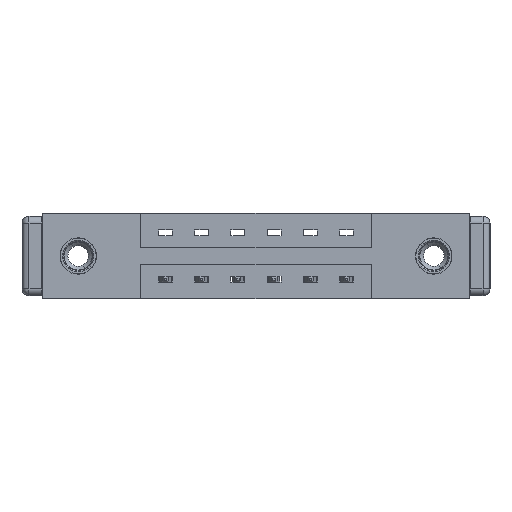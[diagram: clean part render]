
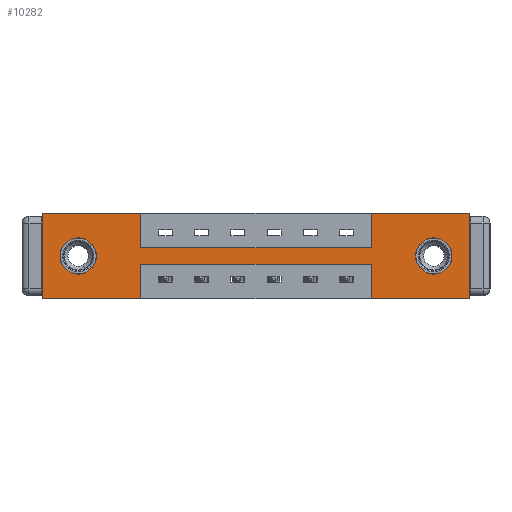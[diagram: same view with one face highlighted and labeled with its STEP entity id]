
A CAD part, front view. The second image highlights one B-rep face of the part: STEP entity #10282.
In plain terms, the highlighted planar face has unit normal (0, -1, 0).
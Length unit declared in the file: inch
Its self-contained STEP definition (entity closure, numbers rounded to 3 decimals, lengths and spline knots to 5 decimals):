
#46 = VERTEX_POINT ( 'NONE', #573 ) ;
#138 = DIRECTION ( 'NONE',  ( 0., -1., 0. ) ) ;
#160 = LINE ( 'NONE', #326, #3913 ) ;
#166 = DIRECTION ( 'NONE',  ( 0., 0., -1. ) ) ;
#237 = DIRECTION ( 'NONE',  ( -1., 0., 0. ) ) ;
#245 = VECTOR ( 'NONE', #1814, 39.37008 ) ;
#326 = CARTESIAN_POINT ( 'NONE',  ( 0.425, 0., 0. ) ) ;
#418 = ORIENTED_EDGE ( 'NONE', *, *, #6473, .F. ) ;
#452 = DIRECTION ( 'NONE',  ( 0., 0., 1. ) ) ;
#557 = VECTOR ( 'NONE', #10802, 39.37008 ) ;
#563 = DIRECTION ( 'NONE',  ( 1., 0., 0. ) ) ;
#570 = FACE_OUTER_BOUND ( 'NONE', #8843, .T. ) ;
#573 = CARTESIAN_POINT ( 'NONE',  ( 1.842, 0., -0.37 ) ) ;
#594 = EDGE_CURVE ( 'NONE', #11487, #4366, #7277, .T. ) ;
#662 = CARTESIAN_POINT ( 'NONE',  ( 1.417, 0., 0. ) ) ;
#727 = LINE ( 'NONE', #2094, #2182 ) ;
#768 = CARTESIAN_POINT ( 'NONE',  ( 0., 0., -0.37 ) ) ;
#1134 = ORIENTED_EDGE ( 'NONE', *, *, #7737, .T. ) ;
#1245 = CARTESIAN_POINT ( 'NONE',  ( 0., 0., -0.37 ) ) ;
#1270 = VERTEX_POINT ( 'NONE', #10253 ) ;
#1301 = CARTESIAN_POINT ( 'NONE',  ( 0.155, 0., -0.107 ) ) ;
#1448 = EDGE_CURVE ( 'NONE', #4177, #11317, #9568, .T. ) ;
#1537 = CIRCLE ( 'NONE', #11228, 0.078 ) ;
#1570 = CARTESIAN_POINT ( 'NONE',  ( 0.155, 0., -0.185 ) ) ;
#1618 = VECTOR ( 'NONE', #10195, 39.37008 ) ;
#1705 = VECTOR ( 'NONE', #9914, 39.37008 ) ;
#1814 = DIRECTION ( 'NONE',  ( 0., 0., -1. ) ) ;
#1933 = DIRECTION ( 'NONE',  ( 1., 0., 0. ) ) ;
#2000 = DIRECTION ( 'NONE',  ( 0., 0., -1. ) ) ;
#2094 = CARTESIAN_POINT ( 'NONE',  ( 0.425, 0., -0.22 ) ) ;
#2120 = EDGE_CURVE ( 'NONE', #9738, #4177, #160, .T. ) ;
#2182 = VECTOR ( 'NONE', #237, 39.37008 ) ;
#2196 = LINE ( 'NONE', #4345, #9953 ) ;
#2490 = DIRECTION ( 'NONE',  ( 0., 1., 0. ) ) ;
#2588 = CARTESIAN_POINT ( 'NONE',  ( 1.417, 0., -0.15 ) ) ;
#2701 = AXIS2_PLACEMENT_3D ( 'NONE', #9938, #4414, #6183 ) ;
#2781 = CARTESIAN_POINT ( 'NONE',  ( 0.425, 0., -0.37 ) ) ;
#2859 = VECTOR ( 'NONE', #11718, 39.37008 ) ;
#2894 = CIRCLE ( 'NONE', #2701, 0.078 ) ;
#2945 = ORIENTED_EDGE ( 'NONE', *, *, #6117, .F. ) ;
#3009 = FACE_BOUND ( 'NONE', #6900, .T. ) ;
#3201 = VERTEX_POINT ( 'NONE', #9277 ) ;
#3442 = EDGE_CURVE ( 'NONE', #6427, #46, #11094, .T. ) ;
#3614 = CARTESIAN_POINT ( 'NONE',  ( 0., 0., 0. ) ) ;
#3913 = VECTOR ( 'NONE', #166, 39.37008 ) ;
#3987 = CARTESIAN_POINT ( 'NONE',  ( 1.417, 0., 0. ) ) ;
#4002 = CARTESIAN_POINT ( 'NONE',  ( 0., 0., -0.37 ) ) ;
#4124 = ORIENTED_EDGE ( 'NONE', *, *, #594, .T. ) ;
#4177 = VERTEX_POINT ( 'NONE', #4698 ) ;
#4199 = ORIENTED_EDGE ( 'NONE', *, *, #7812, .T. ) ;
#4278 = CARTESIAN_POINT ( 'NONE',  ( 0.425, 0., -0.22 ) ) ;
#4290 = CARTESIAN_POINT ( 'NONE',  ( 0.155, 0., -0.185 ) ) ;
#4345 = CARTESIAN_POINT ( 'NONE',  ( 0., 0., 0. ) ) ;
#4366 = VERTEX_POINT ( 'NONE', #5213 ) ;
#4414 = DIRECTION ( 'NONE',  ( 0., 1., 0. ) ) ;
#4698 = CARTESIAN_POINT ( 'NONE',  ( 0.425, 0., -0.15 ) ) ;
#4925 = EDGE_CURVE ( 'NONE', #46, #6889, #5224, .T. ) ;
#4949 = CARTESIAN_POINT ( 'NONE',  ( 0.425, 0., -0.37 ) ) ;
#4983 = VECTOR ( 'NONE', #6867, 39.37008 ) ;
#5023 = EDGE_CURVE ( 'NONE', #8351, #9299, #7412, .T. ) ;
#5213 = CARTESIAN_POINT ( 'NONE',  ( 1.687, 0., -0.107 ) ) ;
#5224 = LINE ( 'NONE', #768, #6534 ) ;
#5279 = CIRCLE ( 'NONE', #10383, 0.078 ) ;
#5541 = CARTESIAN_POINT ( 'NONE',  ( 0.425, 0., 0. ) ) ;
#5774 = ORIENTED_EDGE ( 'NONE', *, *, #7028, .F. ) ;
#5813 = EDGE_CURVE ( 'NONE', #4366, #11487, #2894, .T. ) ;
#5886 = ORIENTED_EDGE ( 'NONE', *, *, #3442, .F. ) ;
#6117 = EDGE_CURVE ( 'NONE', #9299, #9738, #2196, .T. ) ;
#6183 = DIRECTION ( 'NONE',  ( 0., 0., -1. ) ) ;
#6295 = EDGE_CURVE ( 'NONE', #3201, #9210, #727, .T. ) ;
#6316 = LINE ( 'NONE', #662, #1705 ) ;
#6383 = VECTOR ( 'NONE', #8761, 39.37008 ) ;
#6427 = VERTEX_POINT ( 'NONE', #9711 ) ;
#6443 = LINE ( 'NONE', #1245, #4983 ) ;
#6473 = EDGE_CURVE ( 'NONE', #7090, #6427, #10975, .T. ) ;
#6534 = VECTOR ( 'NONE', #8065, 39.37008 ) ;
#6540 = ORIENTED_EDGE ( 'NONE', *, *, #5023, .F. ) ;
#6567 = DIRECTION ( 'NONE',  ( 0., 1., 0. ) ) ;
#6658 = ORIENTED_EDGE ( 'NONE', *, *, #8107, .F. ) ;
#6688 = ORIENTED_EDGE ( 'NONE', *, *, #6295, .F. ) ;
#6783 = ORIENTED_EDGE ( 'NONE', *, *, #4925, .F. ) ;
#6867 = DIRECTION ( 'NONE',  ( -1., 0., 0. ) ) ;
#6889 = VERTEX_POINT ( 'NONE', #10578 ) ;
#6900 = EDGE_LOOP ( 'NONE', ( #4199, #1134 ) ) ;
#6918 = LINE ( 'NONE', #8173, #2859 ) ;
#7028 = EDGE_CURVE ( 'NONE', #11317, #7090, #6316, .T. ) ;
#7090 = VERTEX_POINT ( 'NONE', #3987 ) ;
#7247 = PLANE ( 'NONE',  #9164 ) ;
#7277 = CIRCLE ( 'NONE', #7727, 0.078 ) ;
#7412 = LINE ( 'NONE', #3614, #1618 ) ;
#7420 = DIRECTION ( 'NONE',  ( 0., 0., -1. ) ) ;
#7431 = VERTEX_POINT ( 'NONE', #1301 ) ;
#7483 = EDGE_LOOP ( 'NONE', ( #7534, #4124 ) ) ;
#7534 = ORIENTED_EDGE ( 'NONE', *, *, #5813, .T. ) ;
#7586 = CARTESIAN_POINT ( 'NONE',  ( 1.687, 0., -0.185 ) ) ;
#7622 = LINE ( 'NONE', #2781, #245 ) ;
#7727 = AXIS2_PLACEMENT_3D ( 'NONE', #7586, #6567, #7420 ) ;
#7737 = EDGE_CURVE ( 'NONE', #1270, #7431, #1537, .T. ) ;
#7812 = EDGE_CURVE ( 'NONE', #7431, #1270, #5279, .T. ) ;
#7943 = FACE_BOUND ( 'NONE', #7483, .T. ) ;
#7944 = EDGE_CURVE ( 'NONE', #9210, #9066, #7622, .T. ) ;
#7955 = ORIENTED_EDGE ( 'NONE', *, *, #11309, .F. ) ;
#8065 = DIRECTION ( 'NONE',  ( -1., 0., 0. ) ) ;
#8107 = EDGE_CURVE ( 'NONE', #9066, #8351, #6443, .T. ) ;
#8173 = CARTESIAN_POINT ( 'NONE',  ( 1.417, 0., -0.37 ) ) ;
#8182 = CARTESIAN_POINT ( 'NONE',  ( 0., 0., -0.37 ) ) ;
#8351 = VERTEX_POINT ( 'NONE', #4002 ) ;
#8479 = ORIENTED_EDGE ( 'NONE', *, *, #2120, .F. ) ;
#8485 = ORIENTED_EDGE ( 'NONE', *, *, #1448, .F. ) ;
#8534 = VECTOR ( 'NONE', #1933, 39.37008 ) ;
#8761 = DIRECTION ( 'NONE',  ( 1., 0., 0. ) ) ;
#8843 = EDGE_LOOP ( 'NONE', ( #11844, #6688, #7955, #6783, #5886, #418, #5774, #8485, #8479, #2945, #6540, #6658 ) ) ;
#9066 = VERTEX_POINT ( 'NONE', #4949 ) ;
#9164 = AXIS2_PLACEMENT_3D ( 'NONE', #8182, #138, #2000 ) ;
#9210 = VERTEX_POINT ( 'NONE', #4278 ) ;
#9277 = CARTESIAN_POINT ( 'NONE',  ( 1.417, 0., -0.22 ) ) ;
#9299 = VERTEX_POINT ( 'NONE', #10990 ) ;
#9568 = LINE ( 'NONE', #11471, #6383 ) ;
#9711 = CARTESIAN_POINT ( 'NONE',  ( 1.842, 0., 0. ) ) ;
#9738 = VERTEX_POINT ( 'NONE', #5541 ) ;
#9852 = CARTESIAN_POINT ( 'NONE',  ( 1.842, 0., 0. ) ) ;
#9914 = DIRECTION ( 'NONE',  ( 0., 0., 1. ) ) ;
#9938 = CARTESIAN_POINT ( 'NONE',  ( 1.687, 0., -0.185 ) ) ;
#9953 = VECTOR ( 'NONE', #563, 39.37008 ) ;
#10195 = DIRECTION ( 'NONE',  ( 0., 0., 1. ) ) ;
#10253 = CARTESIAN_POINT ( 'NONE',  ( 0.155, 0., -0.263 ) ) ;
#10282 = ADVANCED_FACE ( 'NONE', ( #7943, #3009, #570 ), #7247, .T. ) ;
#10383 = AXIS2_PLACEMENT_3D ( 'NONE', #1570, #11831, #452 ) ;
#10444 = CARTESIAN_POINT ( 'NONE',  ( 1.687, 0., -0.263 ) ) ;
#10578 = CARTESIAN_POINT ( 'NONE',  ( 1.417, 0., -0.37 ) ) ;
#10802 = DIRECTION ( 'NONE',  ( 0., 0., -1. ) ) ;
#10918 = DIRECTION ( 'NONE',  ( 0., 0., 1. ) ) ;
#10975 = LINE ( 'NONE', #11893, #8534 ) ;
#10990 = CARTESIAN_POINT ( 'NONE',  ( 0., 0., 0. ) ) ;
#11094 = LINE ( 'NONE', #9852, #557 ) ;
#11228 = AXIS2_PLACEMENT_3D ( 'NONE', #4290, #2490, #10918 ) ;
#11309 = EDGE_CURVE ( 'NONE', #6889, #3201, #6918, .T. ) ;
#11317 = VERTEX_POINT ( 'NONE', #2588 ) ;
#11471 = CARTESIAN_POINT ( 'NONE',  ( 0.425, 0., -0.15 ) ) ;
#11487 = VERTEX_POINT ( 'NONE', #10444 ) ;
#11718 = DIRECTION ( 'NONE',  ( 0., 0., 1. ) ) ;
#11831 = DIRECTION ( 'NONE',  ( 0., 1., 0. ) ) ;
#11844 = ORIENTED_EDGE ( 'NONE', *, *, #7944, .F. ) ;
#11893 = CARTESIAN_POINT ( 'NONE',  ( 0., 0., 0. ) ) ;
